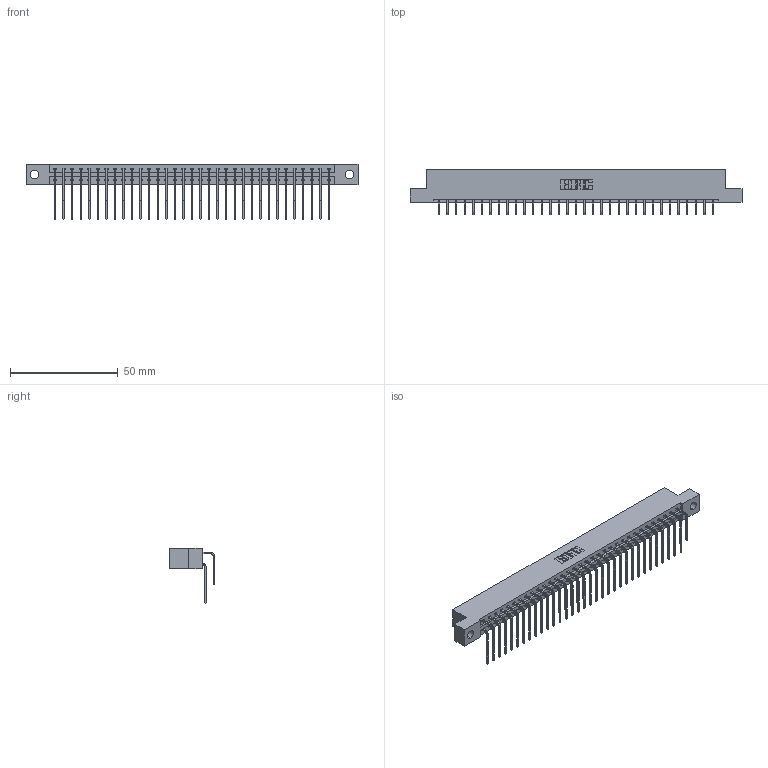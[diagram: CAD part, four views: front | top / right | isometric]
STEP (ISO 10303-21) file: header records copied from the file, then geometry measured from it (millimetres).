
FILE_DESCRIPTION (( 'STEP AP203' ), '1' );
FILE_NAME ('337-066-559-204.STEP', '2018-08-11T08:48:45', ( '' ), ( '' ), 'SwSTEP 2.0', 'SolidWorks 2016', '' );
FILE_SCHEMA (( 'CONFIG_CONTROL_DESIGN' ));
Length unit declared in the file: inch
Products named in the file (4): 345-292-001_558 559 Tail - 1; 345-292-001_559 Tail - 2; 337-066-559-204; 337 Part_Flush Mounting Lugs - 0.156 Dia-TH
Assembly tree (67 placements, depth 2):
  337-066-559-204
    337 Part_Flush Mounting Lugs - 0.156 Dia-TH
    345-292-001_558 559 Tail - 1  x33
    345-292-001_559 Tail - 2  x33
Bounding box: 153.77 x 20.9 x 25.53 mm (x, y, z)
Volume: 16378.7 mm3; surface area: 20137.9 mm2
Topology: 67 solids, 67 shells, 3810 faces, 11333 edges, 7466 vertices
Faces by surface type: plane 2710, cylinder 1100
Entity records: 28537 total; most frequent: CARTESIAN_POINT 4861, ORIENTED_EDGE 4746, DIRECTION 4133, EDGE_CURVE 2373, VECTOR 2205, LINE 2205, VERTEX_POINT 1578, AXIS2_PLACEMENT_3D 964
